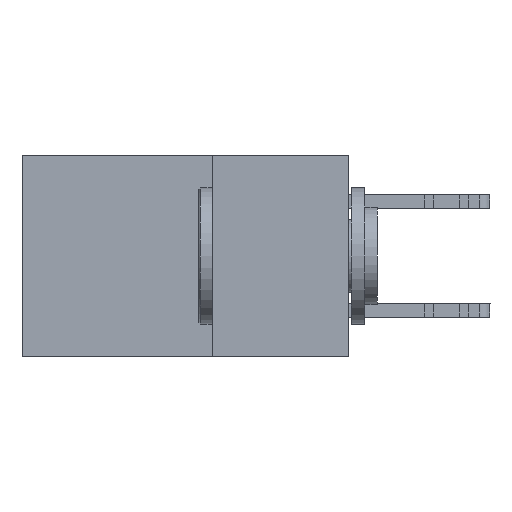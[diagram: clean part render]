
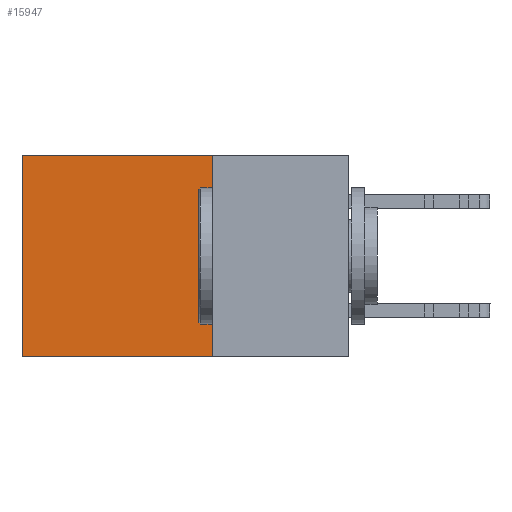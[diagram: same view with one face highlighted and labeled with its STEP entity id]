
A CAD part, left-side view. The second image highlights one B-rep face of the part: STEP entity #15947.
In plain terms, the highlighted planar face has unit normal (-1, 0, 0).
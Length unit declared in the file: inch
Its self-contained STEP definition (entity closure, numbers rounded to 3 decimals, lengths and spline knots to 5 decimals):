
#13 = VECTOR ( 'NONE', #1500, 39.37008 ) ;
#372 = DIRECTION ( 'NONE',  ( 1., 0., 0. ) ) ;
#1001 = LINE ( 'NONE', #27312, #19094 ) ;
#1500 = DIRECTION ( 'NONE',  ( 0., 0., -1. ) ) ;
#1925 = ORIENTED_EDGE ( 'NONE', *, *, #25474, .T. ) ;
#4608 = EDGE_LOOP ( 'NONE', ( #1925, #25505, #24788, #12147 ) ) ;
#6470 = EDGE_CURVE ( 'NONE', #24358, #25475, #12819, .T. ) ;
#8083 = CARTESIAN_POINT ( 'NONE',  ( 0.298, 0.25, 0. ) ) ;
#10692 = FACE_OUTER_BOUND ( 'NONE', #4608, .T. ) ;
#11011 = VECTOR ( 'NONE', #19686, 39.37008 ) ;
#12147 = ORIENTED_EDGE ( 'NONE', *, *, #28435, .T. ) ;
#12819 = LINE ( 'NONE', #8083, #24499 ) ;
#15716 = CARTESIAN_POINT ( 'NONE',  ( 0.298, 0.25, -0.37 ) ) ;
#15947 = ADVANCED_FACE ( 'NONE', ( #10692 ), #26285, .F. ) ;
#16970 = DIRECTION ( 'NONE',  ( 0., 0., -1. ) ) ;
#17390 = CARTESIAN_POINT ( 'NONE',  ( 0.298, 0.25, 0. ) ) ;
#18193 = LINE ( 'NONE', #29761, #13 ) ;
#19094 = VECTOR ( 'NONE', #29671, 39.37008 ) ;
#19177 = CARTESIAN_POINT ( 'NONE',  ( 0.298, 0.25, 0. ) ) ;
#19686 = DIRECTION ( 'NONE',  ( 0., 1., 0. ) ) ;
#19939 = VERTEX_POINT ( 'NONE', #25444 ) ;
#21763 = EDGE_CURVE ( 'NONE', #25475, #19939, #1001, .T. ) ;
#22028 = DIRECTION ( 'NONE',  ( 0., 0., -1. ) ) ;
#23412 = LINE ( 'NONE', #17390, #11011 ) ;
#23627 = CARTESIAN_POINT ( 'NONE',  ( 0.298, 0.25, 0. ) ) ;
#24358 = VERTEX_POINT ( 'NONE', #23627 ) ;
#24499 = VECTOR ( 'NONE', #22028, 39.37008 ) ;
#24788 = ORIENTED_EDGE ( 'NONE', *, *, #6470, .F. ) ;
#25444 = CARTESIAN_POINT ( 'NONE',  ( 0.298, 0.6, -0.37 ) ) ;
#25474 = EDGE_CURVE ( 'NONE', #27918, #19939, #18193, .T. ) ;
#25475 = VERTEX_POINT ( 'NONE', #15716 ) ;
#25505 = ORIENTED_EDGE ( 'NONE', *, *, #21763, .F. ) ;
#26285 = PLANE ( 'NONE',  #28886 ) ;
#27312 = CARTESIAN_POINT ( 'NONE',  ( 0.298, 0.25, -0.37 ) ) ;
#27918 = VERTEX_POINT ( 'NONE', #29627 ) ;
#28435 = EDGE_CURVE ( 'NONE', #24358, #27918, #23412, .T. ) ;
#28886 = AXIS2_PLACEMENT_3D ( 'NONE', #19177, #372, #16970 ) ;
#29627 = CARTESIAN_POINT ( 'NONE',  ( 0.298, 0.6, 0. ) ) ;
#29671 = DIRECTION ( 'NONE',  ( 0., 1., 0. ) ) ;
#29761 = CARTESIAN_POINT ( 'NONE',  ( 0.298, 0.6, 0. ) ) ;
